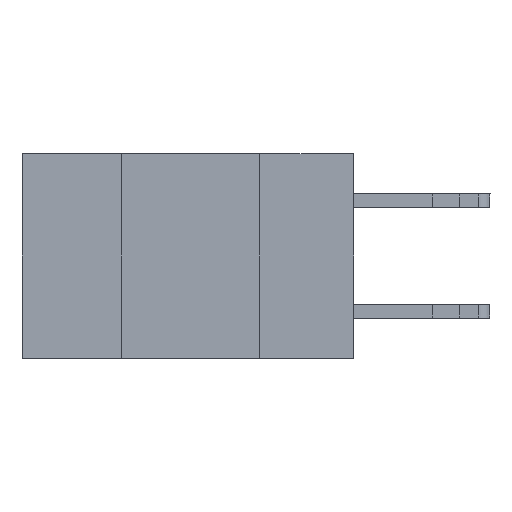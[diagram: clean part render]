
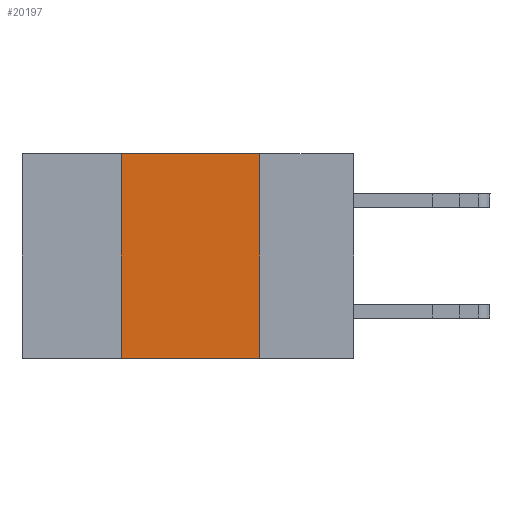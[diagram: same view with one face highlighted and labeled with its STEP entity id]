
A CAD part, left-side view. The second image highlights one B-rep face of the part: STEP entity #20197.
In plain terms, the highlighted planar face has unit normal (-1, 0, 0).
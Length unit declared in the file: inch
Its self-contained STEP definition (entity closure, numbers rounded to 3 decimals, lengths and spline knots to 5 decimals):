
#1648 = VERTEX_POINT ( 'NONE', #7064 ) ;
#1775 = VECTOR ( 'NONE', #6960, 39.37008 ) ;
#2839 = EDGE_CURVE ( 'NONE', #10172, #17803, #22538, .T. ) ;
#3191 = EDGE_LOOP ( 'NONE', ( #7331, #18854, #17866, #15977 ) ) ;
#3507 = EDGE_CURVE ( 'NONE', #22369, #10172, #11144, .T. ) ;
#3758 = DIRECTION ( 'NONE',  ( 0., 0., 1. ) ) ;
#3771 = DIRECTION ( 'NONE',  ( 0., -1., 0. ) ) ;
#4088 = CARTESIAN_POINT ( 'NONE',  ( 0., 0.17, 0. ) ) ;
#4625 = EDGE_CURVE ( 'NONE', #1648, #17803, #6725, .T. ) ;
#5031 = VECTOR ( 'NONE', #3771, 39.37008 ) ;
#6725 = LINE ( 'NONE', #15836, #1775 ) ;
#6960 = DIRECTION ( 'NONE',  ( 0., -1., 0. ) ) ;
#7024 = CARTESIAN_POINT ( 'NONE',  ( 0., 0.42, 0. ) ) ;
#7064 = CARTESIAN_POINT ( 'NONE',  ( 0., 0.42, -0.37 ) ) ;
#7331 = ORIENTED_EDGE ( 'NONE', *, *, #2839, .F. ) ;
#8400 = DIRECTION ( 'NONE',  ( 0., 0., -1. ) ) ;
#9634 = EDGE_CURVE ( 'NONE', #1648, #22369, #20360, .T. ) ;
#9870 = CARTESIAN_POINT ( 'NONE',  ( 0., 0.6, 0. ) ) ;
#10172 = VERTEX_POINT ( 'NONE', #4088 ) ;
#11144 = LINE ( 'NONE', #22569, #5031 ) ;
#11255 = AXIS2_PLACEMENT_3D ( 'NONE', #9870, #17396, #8400 ) ;
#11955 = VECTOR ( 'NONE', #13328, 39.37008 ) ;
#13328 = DIRECTION ( 'NONE',  ( 0., 0., -1. ) ) ;
#13765 = PLANE ( 'NONE',  #11255 ) ;
#14678 = VECTOR ( 'NONE', #3758, 39.37008 ) ;
#15151 = CARTESIAN_POINT ( 'NONE',  ( 0., 0.17, 0. ) ) ;
#15578 = FACE_OUTER_BOUND ( 'NONE', #3191, .T. ) ;
#15836 = CARTESIAN_POINT ( 'NONE',  ( 0., 0.6, -0.37 ) ) ;
#15977 = ORIENTED_EDGE ( 'NONE', *, *, #4625, .T. ) ;
#17396 = DIRECTION ( 'NONE',  ( 1., 0., 0. ) ) ;
#17803 = VERTEX_POINT ( 'NONE', #21200 ) ;
#17866 = ORIENTED_EDGE ( 'NONE', *, *, #9634, .F. ) ;
#18854 = ORIENTED_EDGE ( 'NONE', *, *, #3507, .F. ) ;
#20197 = ADVANCED_FACE ( 'NONE', ( #15578 ), #13765, .F. ) ;
#20360 = LINE ( 'NONE', #7024, #14678 ) ;
#21200 = CARTESIAN_POINT ( 'NONE',  ( 0., 0.17, -0.37 ) ) ;
#21727 = CARTESIAN_POINT ( 'NONE',  ( 0., 0.42, 0. ) ) ;
#22369 = VERTEX_POINT ( 'NONE', #21727 ) ;
#22538 = LINE ( 'NONE', #15151, #11955 ) ;
#22569 = CARTESIAN_POINT ( 'NONE',  ( 0., 0.6, 0. ) ) ;
